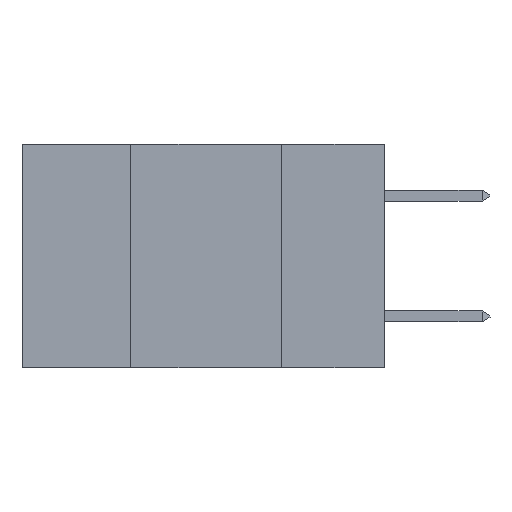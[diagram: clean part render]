
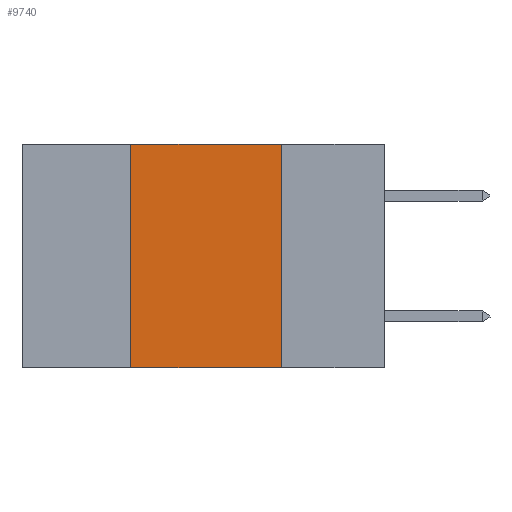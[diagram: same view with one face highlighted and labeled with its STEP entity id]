
A CAD part, left-side view. The second image highlights one B-rep face of the part: STEP entity #9740.
In plain terms, the highlighted planar face has unit normal (-1, 0, 0).
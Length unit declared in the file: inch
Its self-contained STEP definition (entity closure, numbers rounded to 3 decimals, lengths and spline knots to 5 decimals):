
#118 = CARTESIAN_POINT ( 'NONE',  ( 0., 0.42, -0.37 ) ) ;
#471 = VERTEX_POINT ( 'NONE', #1196 ) ;
#856 = FACE_OUTER_BOUND ( 'NONE', #4207, .T. ) ;
#1196 = CARTESIAN_POINT ( 'NONE',  ( 0., 0.17, 0. ) ) ;
#1330 = EDGE_CURVE ( 'NONE', #3328, #20890, #3935, .T. ) ;
#1415 = VERTEX_POINT ( 'NONE', #6987 ) ;
#2309 = EDGE_CURVE ( 'NONE', #471, #1415, #13932, .T. ) ;
#2520 = CARTESIAN_POINT ( 'NONE',  ( 0., 0.6, 0. ) ) ;
#3162 = DIRECTION ( 'NONE',  ( 0., -1., 0. ) ) ;
#3328 = VERTEX_POINT ( 'NONE', #118 ) ;
#3404 = VECTOR ( 'NONE', #8441, 39.37008 ) ;
#3706 = CARTESIAN_POINT ( 'NONE',  ( 0., 0.42, 0. ) ) ;
#3935 = LINE ( 'NONE', #3706, #3404 ) ;
#4203 = DIRECTION ( 'NONE',  ( 0., 0., -1. ) ) ;
#4207 = EDGE_LOOP ( 'NONE', ( #17118, #17263, #8292, #19520 ) ) ;
#5164 = VECTOR ( 'NONE', #15808, 39.37008 ) ;
#5789 = LINE ( 'NONE', #14728, #13498 ) ;
#5899 = CARTESIAN_POINT ( 'NONE',  ( 0., 0.17, 0. ) ) ;
#6987 = CARTESIAN_POINT ( 'NONE',  ( 0., 0.17, -0.37 ) ) ;
#8292 = ORIENTED_EDGE ( 'NONE', *, *, #1330, .F. ) ;
#8441 = DIRECTION ( 'NONE',  ( 0., 0., 1. ) ) ;
#9740 = ADVANCED_FACE ( 'NONE', ( #856 ), #20659, .F. ) ;
#10516 = EDGE_CURVE ( 'NONE', #20890, #471, #11667, .T. ) ;
#11667 = LINE ( 'NONE', #19613, #19978 ) ;
#13498 = VECTOR ( 'NONE', #3162, 39.37008 ) ;
#13932 = LINE ( 'NONE', #5899, #5164 ) ;
#14077 = DIRECTION ( 'NONE',  ( 1., 0., 0. ) ) ;
#14728 = CARTESIAN_POINT ( 'NONE',  ( 0., 0.6, -0.37 ) ) ;
#15808 = DIRECTION ( 'NONE',  ( 0., 0., -1. ) ) ;
#16769 = CARTESIAN_POINT ( 'NONE',  ( 0., 0.42, 0. ) ) ;
#17118 = ORIENTED_EDGE ( 'NONE', *, *, #2309, .F. ) ;
#17263 = ORIENTED_EDGE ( 'NONE', *, *, #10516, .F. ) ;
#18555 = EDGE_CURVE ( 'NONE', #3328, #1415, #5789, .T. ) ;
#19520 = ORIENTED_EDGE ( 'NONE', *, *, #18555, .T. ) ;
#19596 = AXIS2_PLACEMENT_3D ( 'NONE', #2520, #14077, #4203 ) ;
#19613 = CARTESIAN_POINT ( 'NONE',  ( 0., 0.6, 0. ) ) ;
#19978 = VECTOR ( 'NONE', #21260, 39.37008 ) ;
#20659 = PLANE ( 'NONE',  #19596 ) ;
#20890 = VERTEX_POINT ( 'NONE', #16769 ) ;
#21260 = DIRECTION ( 'NONE',  ( 0., -1., 0. ) ) ;
